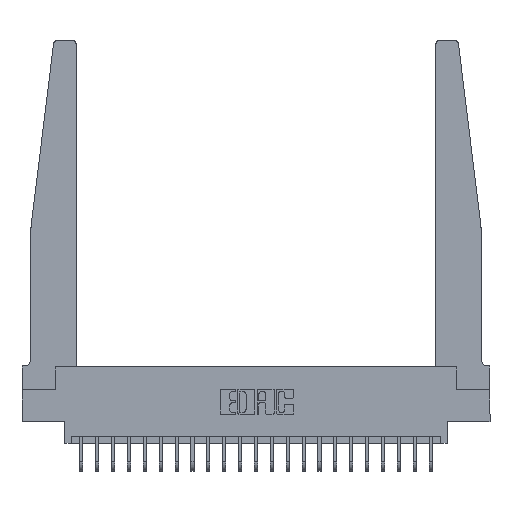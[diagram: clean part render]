
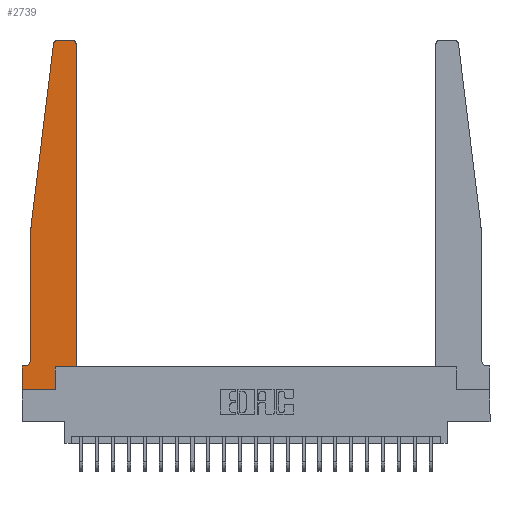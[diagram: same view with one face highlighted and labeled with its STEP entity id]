
A CAD part, top view. The second image highlights one B-rep face of the part: STEP entity #2739.
In plain terms, the highlighted planar face has unit normal (0, 0, 1).
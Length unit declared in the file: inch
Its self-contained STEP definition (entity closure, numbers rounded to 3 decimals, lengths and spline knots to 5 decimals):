
#293 = FACE_OUTER_BOUND ( 'NONE', #6091, .T. ) ;
#327 = ORIENTED_EDGE ( 'NONE', *, *, #4285, .T. ) ;
#358 = VECTOR ( 'NONE', #9531, 39.37008 ) ;
#1277 = VECTOR ( 'NONE', #15625, 39.37008 ) ;
#1637 = VECTOR ( 'NONE', #18589, 39.37008 ) ;
#1782 = LINE ( 'NONE', #13003, #18224 ) ;
#2045 = CARTESIAN_POINT ( 'NONE',  ( 0.065, 1.25, 0.37 ) ) ;
#2496 = LINE ( 'NONE', #14528, #3664 ) ;
#2739 = ADVANCED_FACE ( 'NONE', ( #293 ), #5531, .T. ) ;
#2979 = CARTESIAN_POINT ( 'NONE',  ( 0.425, 0.18, 0.37 ) ) ;
#3212 = VERTEX_POINT ( 'NONE', #2979 ) ;
#3298 = DIRECTION ( 'NONE',  ( -1., 0., 0. ) ) ;
#3664 = VECTOR ( 'NONE', #3298, 39.37008 ) ;
#3842 = DIRECTION ( 'NONE',  ( 0., -1., 0. ) ) ;
#3912 = VECTOR ( 'NONE', #3842, 39.37008 ) ;
#4052 = CARTESIAN_POINT ( 'NONE',  ( 0., 0.1875, 0.37 ) ) ;
#4056 = VERTEX_POINT ( 'NONE', #6011 ) ;
#4116 = EDGE_CURVE ( 'NONE', #12933, #20070, #10455, .T. ) ;
#4200 = AXIS2_PLACEMENT_3D ( 'NONE', #24170, #13070, #16545 ) ;
#4263 = CARTESIAN_POINT ( 'NONE',  ( 0.015, 0.2375, 0.37 ) ) ;
#4285 = EDGE_CURVE ( 'NONE', #11533, #3212, #16653, .T. ) ;
#4501 = DIRECTION ( 'NONE',  ( 0., 0., -1. ) ) ;
#4878 = VECTOR ( 'NONE', #12485, 39.37008 ) ;
#5531 = PLANE ( 'NONE',  #4200 ) ;
#5769 = CARTESIAN_POINT ( 'NONE',  ( 0.395, 2.75, 0.37 ) ) ;
#5948 = LINE ( 'NONE', #18491, #1277 ) ;
#5998 = EDGE_CURVE ( 'NONE', #7079, #6107, #6570, .T. ) ;
#6011 = CARTESIAN_POINT ( 'NONE',  ( 0.065, 0.2375, 0.37 ) ) ;
#6091 = EDGE_LOOP ( 'NONE', ( #17008, #17913, #9030, #19031, #11024, #11712, #20441, #17577, #19337, #327, #8129, #7358 ) ) ;
#6107 = VERTEX_POINT ( 'NONE', #19704 ) ;
#6270 = VERTEX_POINT ( 'NONE', #14181 ) ;
#6570 = LINE ( 'NONE', #18659, #3912 ) ;
#6844 = CARTESIAN_POINT ( 'NONE',  ( 0.2605, 0.18, 0.37 ) ) ;
#6916 = CIRCLE ( 'NONE', #22237, 0.05 ) ;
#7059 = EDGE_CURVE ( 'NONE', #20070, #4056, #22991, .T. ) ;
#7079 = VERTEX_POINT ( 'NONE', #4052 ) ;
#7287 = CARTESIAN_POINT ( 'NONE',  ( 0.015, 0.1875, 0.37 ) ) ;
#7358 = ORIENTED_EDGE ( 'NONE', *, *, #10349, .T. ) ;
#7515 = DIRECTION ( 'NONE',  ( -1., 0., 0. ) ) ;
#7875 = VERTEX_POINT ( 'NONE', #8140 ) ;
#8035 = VECTOR ( 'NONE', #21973, 39.37008 ) ;
#8129 = ORIENTED_EDGE ( 'NONE', *, *, #19973, .T. ) ;
#8140 = CARTESIAN_POINT ( 'NONE',  ( 0.425, 2.72, 0.37 ) ) ;
#8266 = CIRCLE ( 'NONE', #17981, 0.03 ) ;
#9030 = ORIENTED_EDGE ( 'NONE', *, *, #4116, .T. ) ;
#9037 = DIRECTION ( 'NONE',  ( 1., 0., 0. ) ) ;
#9469 = LINE ( 'NONE', #6844, #8035 ) ;
#9531 = DIRECTION ( 'NONE',  ( 0., -1., 0. ) ) ;
#10349 = EDGE_CURVE ( 'NONE', #7875, #23111, #23581, .T. ) ;
#10455 = LINE ( 'NONE', #16193, #4878 ) ;
#11024 = ORIENTED_EDGE ( 'NONE', *, *, #17447, .T. ) ;
#11533 = VERTEX_POINT ( 'NONE', #16360 ) ;
#11668 = CARTESIAN_POINT ( 'NONE',  ( 0.065, 1.25, 0.37 ) ) ;
#11712 = ORIENTED_EDGE ( 'NONE', *, *, #17823, .T. ) ;
#11977 = CARTESIAN_POINT ( 'NONE',  ( 0.425, 0.18, 0.37 ) ) ;
#12485 = DIRECTION ( 'NONE',  ( -0.122, -0.992, 0. ) ) ;
#12507 = CARTESIAN_POINT ( 'NONE',  ( 0.24675, 2.72367, 0.37 ) ) ;
#12722 = DIRECTION ( 'NONE',  ( 0., 0., 1. ) ) ;
#12933 = VERTEX_POINT ( 'NONE', #12507 ) ;
#13003 = CARTESIAN_POINT ( 'NONE',  ( 0.25, 2.75, 0.37 ) ) ;
#13070 = DIRECTION ( 'NONE',  ( 0., 0., 1. ) ) ;
#14181 = CARTESIAN_POINT ( 'NONE',  ( 0.2605, 0., 0.37 ) ) ;
#14528 = CARTESIAN_POINT ( 'NONE',  ( 0.065, 0.1875, 0.37 ) ) ;
#14864 = VERTEX_POINT ( 'NONE', #7287 ) ;
#14996 = EDGE_CURVE ( 'NONE', #23111, #23412, #1782, .T. ) ;
#15017 = DIRECTION ( 'NONE',  ( 0., 0., 1. ) ) ;
#15099 = LINE ( 'NONE', #16688, #1637 ) ;
#15625 = DIRECTION ( 'NONE',  ( 0., 1., 0. ) ) ;
#15763 = DIRECTION ( 'NONE',  ( -1., 0., 0. ) ) ;
#16193 = CARTESIAN_POINT ( 'NONE',  ( 0.065, 1.25, 0.37 ) ) ;
#16360 = CARTESIAN_POINT ( 'NONE',  ( 0.2605, 0.18, 0.37 ) ) ;
#16545 = DIRECTION ( 'NONE',  ( 1., 0., 0. ) ) ;
#16653 = LINE ( 'NONE', #11977, #24278 ) ;
#16688 = CARTESIAN_POINT ( 'NONE',  ( 0., 0., 0.37 ) ) ;
#17008 = ORIENTED_EDGE ( 'NONE', *, *, #14996, .T. ) ;
#17447 = EDGE_CURVE ( 'NONE', #4056, #14864, #6916, .T. ) ;
#17577 = ORIENTED_EDGE ( 'NONE', *, *, #22253, .T. ) ;
#17823 = EDGE_CURVE ( 'NONE', #14864, #7079, #2496, .T. ) ;
#17877 = AXIS2_PLACEMENT_3D ( 'NONE', #18721, #15017, #18875 ) ;
#17913 = ORIENTED_EDGE ( 'NONE', *, *, #20413, .T. ) ;
#17981 = AXIS2_PLACEMENT_3D ( 'NONE', #18271, #12722, #9037 ) ;
#18224 = VECTOR ( 'NONE', #7515, 39.37008 ) ;
#18271 = CARTESIAN_POINT ( 'NONE',  ( 0.27653, 2.72, 0.37 ) ) ;
#18491 = CARTESIAN_POINT ( 'NONE',  ( 0.425, 0.18, 0.37 ) ) ;
#18589 = DIRECTION ( 'NONE',  ( 1., 0., 0. ) ) ;
#18659 = CARTESIAN_POINT ( 'NONE',  ( 0., 0., 0.37 ) ) ;
#18721 = CARTESIAN_POINT ( 'NONE',  ( 0.395, 2.72, 0.37 ) ) ;
#18875 = DIRECTION ( 'NONE',  ( 1., 0., 0. ) ) ;
#19031 = ORIENTED_EDGE ( 'NONE', *, *, #7059, .T. ) ;
#19168 = EDGE_CURVE ( 'NONE', #6270, #11533, #9469, .T. ) ;
#19337 = ORIENTED_EDGE ( 'NONE', *, *, #19168, .T. ) ;
#19704 = CARTESIAN_POINT ( 'NONE',  ( 0., 0., 0.37 ) ) ;
#19973 = EDGE_CURVE ( 'NONE', #3212, #7875, #5948, .T. ) ;
#20070 = VERTEX_POINT ( 'NONE', #11668 ) ;
#20413 = EDGE_CURVE ( 'NONE', #23412, #12933, #8266, .T. ) ;
#20441 = ORIENTED_EDGE ( 'NONE', *, *, #5998, .T. ) ;
#21973 = DIRECTION ( 'NONE',  ( 0., 1., 0. ) ) ;
#22237 = AXIS2_PLACEMENT_3D ( 'NONE', #4263, #4501, #15763 ) ;
#22253 = EDGE_CURVE ( 'NONE', #6107, #6270, #15099, .T. ) ;
#22991 = LINE ( 'NONE', #2045, #358 ) ;
#23111 = VERTEX_POINT ( 'NONE', #5769 ) ;
#23255 = DIRECTION ( 'NONE',  ( 1., 0., 0. ) ) ;
#23412 = VERTEX_POINT ( 'NONE', #24162 ) ;
#23581 = CIRCLE ( 'NONE', #17877, 0.03 ) ;
#24162 = CARTESIAN_POINT ( 'NONE',  ( 0.27653, 2.75, 0.37 ) ) ;
#24170 = CARTESIAN_POINT ( 'NONE',  ( 0., 0.1875, 0.37 ) ) ;
#24278 = VECTOR ( 'NONE', #23255, 39.37008 ) ;
